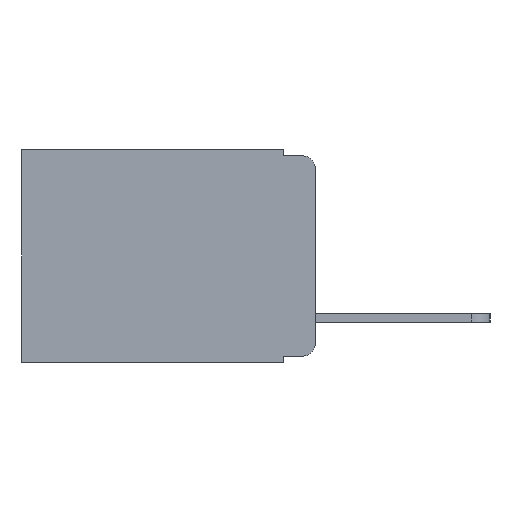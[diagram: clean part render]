
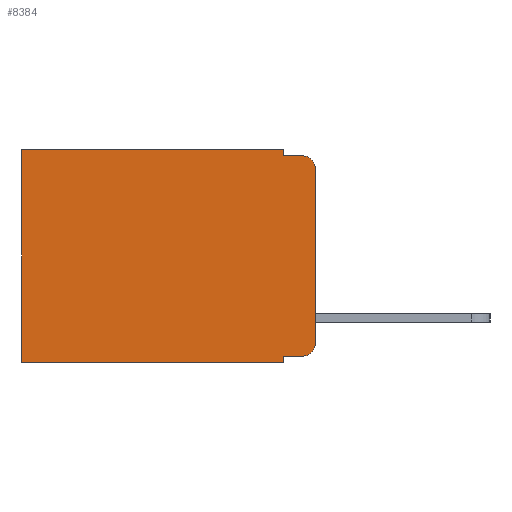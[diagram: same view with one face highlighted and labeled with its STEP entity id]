
A CAD part, left-side view. The second image highlights one B-rep face of the part: STEP entity #8384.
In plain terms, the highlighted planar face has unit normal (-1, 0, 0).
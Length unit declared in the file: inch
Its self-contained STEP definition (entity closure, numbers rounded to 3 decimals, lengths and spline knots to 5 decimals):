
#4 = AXIS2_PLACEMENT_3D ( 'NONE', #12230, #14070, #2798 ) ;
#23 = LINE ( 'NONE', #3333, #4672 ) ;
#144 = EDGE_CURVE ( 'NONE', #23648, #16592, #9002, .T. ) ;
#603 = CARTESIAN_POINT ( 'NONE',  ( 0.298, 0.051, -0.333 ) ) ;
#751 = DIRECTION ( 'NONE',  ( 0., 0., -1. ) ) ;
#809 = CARTESIAN_POINT ( 'NONE',  ( 0.298, 0.02, -0.313 ) ) ;
#862 = DIRECTION ( 'NONE',  ( 0., 0., -1. ) ) ;
#2124 = AXIS2_PLACEMENT_3D ( 'NONE', #6966, #5714, #5521 ) ;
#2798 = DIRECTION ( 'NONE',  ( 0., 0., -1. ) ) ;
#2810 = DIRECTION ( 'NONE',  ( 0., 0., -1. ) ) ;
#2841 = CARTESIAN_POINT ( 'NONE',  ( 0.298, 0.051, -0.01 ) ) ;
#2900 = EDGE_CURVE ( 'NONE', #4790, #19583, #23, .T. ) ;
#2984 = VECTOR ( 'NONE', #9219, 39.37008 ) ;
#3263 = CARTESIAN_POINT ( 'NONE',  ( 0.298, 0.051, -0.333 ) ) ;
#3333 = CARTESIAN_POINT ( 'NONE',  ( 0.298, 0.051, 0. ) ) ;
#3474 = ORIENTED_EDGE ( 'NONE', *, *, #17270, .T. ) ;
#4129 = CARTESIAN_POINT ( 'NONE',  ( 0.298, 0.051, 0. ) ) ;
#4145 = EDGE_CURVE ( 'NONE', #23648, #5442, #12527, .T. ) ;
#4156 = DIRECTION ( 'NONE',  ( 0., 0., -1. ) ) ;
#4388 = ORIENTED_EDGE ( 'NONE', *, *, #19689, .F. ) ;
#4473 = AXIS2_PLACEMENT_3D ( 'NONE', #809, #14085, #2810 ) ;
#4602 = VERTEX_POINT ( 'NONE', #4717 ) ;
#4672 = VECTOR ( 'NONE', #4156, 39.37008 ) ;
#4717 = CARTESIAN_POINT ( 'NONE',  ( 0.298, 0.02, -0.333 ) ) ;
#4790 = VERTEX_POINT ( 'NONE', #3263 ) ;
#5396 = CARTESIAN_POINT ( 'NONE',  ( 0.298, 0.051, -0.01 ) ) ;
#5442 = VERTEX_POINT ( 'NONE', #18553 ) ;
#5521 = DIRECTION ( 'NONE',  ( 0., 0., -1. ) ) ;
#5605 = ORIENTED_EDGE ( 'NONE', *, *, #6215, .F. ) ;
#5714 = DIRECTION ( 'NONE',  ( -1., 0., 0. ) ) ;
#5974 = CARTESIAN_POINT ( 'NONE',  ( 0.298, 0., 0. ) ) ;
#6215 = EDGE_CURVE ( 'NONE', #19583, #13691, #21770, .T. ) ;
#6833 = EDGE_CURVE ( 'NONE', #11053, #19114, #18230, .T. ) ;
#6944 = VECTOR ( 'NONE', #11579, 39.37008 ) ;
#6966 = CARTESIAN_POINT ( 'NONE',  ( 0.298, 0.02, -0.03 ) ) ;
#7774 = CARTESIAN_POINT ( 'NONE',  ( 0.298, 0.473, -0.343 ) ) ;
#7918 = CARTESIAN_POINT ( 'NONE',  ( 0.298, 0., -0.343 ) ) ;
#8384 = ADVANCED_FACE ( 'NONE', ( #18670 ), #10410, .F. ) ;
#8412 = VECTOR ( 'NONE', #17088, 39.37008 ) ;
#8932 = CARTESIAN_POINT ( 'NONE',  ( 0.298, 0., 0. ) ) ;
#9002 = LINE ( 'NONE', #8932, #23217 ) ;
#9219 = DIRECTION ( 'NONE',  ( 0., -1., 0. ) ) ;
#9836 = VECTOR ( 'NONE', #751, 39.37008 ) ;
#10375 = CARTESIAN_POINT ( 'NONE',  ( 0.298, 0.473, 0. ) ) ;
#10410 = PLANE ( 'NONE',  #4 ) ;
#10588 = EDGE_CURVE ( 'NONE', #4790, #4602, #21174, .T. ) ;
#11053 = VERTEX_POINT ( 'NONE', #4129 ) ;
#11216 = ORIENTED_EDGE ( 'NONE', *, *, #10588, .T. ) ;
#11579 = DIRECTION ( 'NONE',  ( 0., 1., 0. ) ) ;
#11767 = ORIENTED_EDGE ( 'NONE', *, *, #2900, .F. ) ;
#12023 = ORIENTED_EDGE ( 'NONE', *, *, #4145, .T. ) ;
#12056 = DIRECTION ( 'NONE',  ( 0., -1., 0. ) ) ;
#12230 = CARTESIAN_POINT ( 'NONE',  ( 0.298, 0., 0. ) ) ;
#12527 = CIRCLE ( 'NONE', #2124, 0.02 ) ;
#12764 = VERTEX_POINT ( 'NONE', #2841 ) ;
#12955 = EDGE_CURVE ( 'NONE', #12764, #5442, #13025, .T. ) ;
#13025 = LINE ( 'NONE', #5396, #2984 ) ;
#13691 = VERTEX_POINT ( 'NONE', #7774 ) ;
#14070 = DIRECTION ( 'NONE',  ( 1., 0., 0. ) ) ;
#14085 = DIRECTION ( 'NONE',  ( -1., 0., 0. ) ) ;
#15316 = CIRCLE ( 'NONE', #4473, 0.02 ) ;
#15635 = VECTOR ( 'NONE', #12056, 39.37008 ) ;
#15999 = CARTESIAN_POINT ( 'NONE',  ( 0.298, 0.051, 0. ) ) ;
#16592 = VERTEX_POINT ( 'NONE', #23181 ) ;
#17088 = DIRECTION ( 'NONE',  ( 0., 1., 0. ) ) ;
#17255 = ORIENTED_EDGE ( 'NONE', *, *, #18419, .T. ) ;
#17270 = EDGE_CURVE ( 'NONE', #4602, #16592, #15316, .T. ) ;
#17512 = DIRECTION ( 'NONE',  ( 0., 0., -1. ) ) ;
#17896 = CARTESIAN_POINT ( 'NONE',  ( 0.298, 0.473, 0. ) ) ;
#18230 = LINE ( 'NONE', #5974, #8412 ) ;
#18419 = EDGE_CURVE ( 'NONE', #19114, #13691, #19631, .T. ) ;
#18553 = CARTESIAN_POINT ( 'NONE',  ( 0.298, 0.02, -0.01 ) ) ;
#18670 = FACE_OUTER_BOUND ( 'NONE', #20907, .T. ) ;
#18998 = VECTOR ( 'NONE', #862, 39.37008 ) ;
#19114 = VERTEX_POINT ( 'NONE', #17896 ) ;
#19540 = ORIENTED_EDGE ( 'NONE', *, *, #144, .F. ) ;
#19566 = LINE ( 'NONE', #15999, #18998 ) ;
#19583 = VERTEX_POINT ( 'NONE', #23124 ) ;
#19631 = LINE ( 'NONE', #10375, #9836 ) ;
#19689 = EDGE_CURVE ( 'NONE', #11053, #12764, #19566, .T. ) ;
#20431 = CARTESIAN_POINT ( 'NONE',  ( 0.298, 0., -0.03 ) ) ;
#20720 = ORIENTED_EDGE ( 'NONE', *, *, #12955, .F. ) ;
#20907 = EDGE_LOOP ( 'NONE', ( #19540, #12023, #20720, #4388, #24268, #17255, #5605, #11767, #11216, #3474 ) ) ;
#21174 = LINE ( 'NONE', #603, #15635 ) ;
#21770 = LINE ( 'NONE', #7918, #6944 ) ;
#23124 = CARTESIAN_POINT ( 'NONE',  ( 0.298, 0.051, -0.343 ) ) ;
#23181 = CARTESIAN_POINT ( 'NONE',  ( 0.298, 0., -0.313 ) ) ;
#23217 = VECTOR ( 'NONE', #17512, 39.37008 ) ;
#23648 = VERTEX_POINT ( 'NONE', #20431 ) ;
#24268 = ORIENTED_EDGE ( 'NONE', *, *, #6833, .T. ) ;
